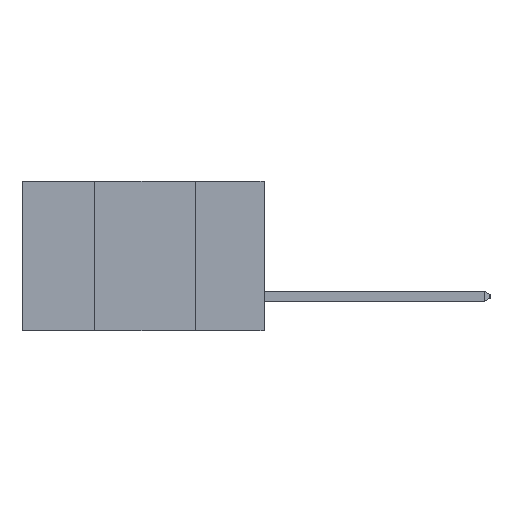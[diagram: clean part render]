
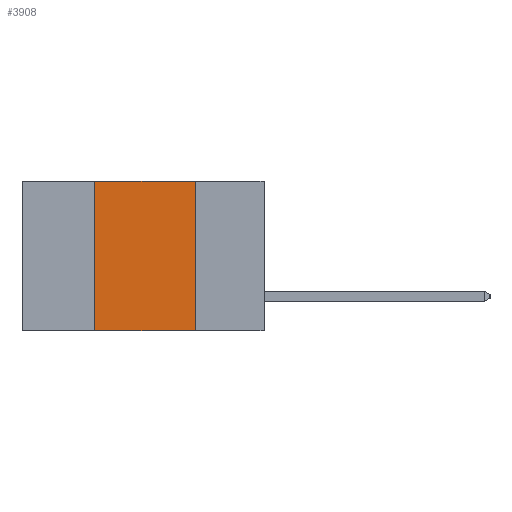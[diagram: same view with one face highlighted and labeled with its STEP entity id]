
A CAD part, left-side view. The second image highlights one B-rep face of the part: STEP entity #3908.
In plain terms, the highlighted planar face has unit normal (-1, 0, 0).
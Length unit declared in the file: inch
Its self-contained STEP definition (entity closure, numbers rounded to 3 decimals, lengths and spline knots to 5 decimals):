
#106 = CARTESIAN_POINT ( 'NONE',  ( 0., 0.6, -0.37 ) ) ;
#1495 = EDGE_LOOP ( 'NONE', ( #17972, #2869, #17055, #5556 ) ) ;
#1849 = CARTESIAN_POINT ( 'NONE',  ( 0., 0.17, 0. ) ) ;
#2804 = VECTOR ( 'NONE', #8386, 39.37008 ) ;
#2869 = ORIENTED_EDGE ( 'NONE', *, *, #15833, .F. ) ;
#3908 = ADVANCED_FACE ( 'NONE', ( #11621 ), #4209, .F. ) ;
#3989 = AXIS2_PLACEMENT_3D ( 'NONE', #4275, #4074, #4058 ) ;
#4058 = DIRECTION ( 'NONE',  ( 0., 0., -1. ) ) ;
#4074 = DIRECTION ( 'NONE',  ( 1., 0., 0. ) ) ;
#4209 = PLANE ( 'NONE',  #3989 ) ;
#4275 = CARTESIAN_POINT ( 'NONE',  ( 0., 0.6, 0. ) ) ;
#4342 = DIRECTION ( 'NONE',  ( 0., 0., 1. ) ) ;
#4562 = EDGE_CURVE ( 'NONE', #18565, #7516, #11821, .T. ) ;
#4950 = VERTEX_POINT ( 'NONE', #15550 ) ;
#5010 = CARTESIAN_POINT ( 'NONE',  ( 0., 0.42, -0.37 ) ) ;
#5436 = CARTESIAN_POINT ( 'NONE',  ( 0., 0.42, -0.37 ) ) ;
#5556 = ORIENTED_EDGE ( 'NONE', *, *, #16079, .T. ) ;
#7516 = VERTEX_POINT ( 'NONE', #8032 ) ;
#8032 = CARTESIAN_POINT ( 'NONE',  ( 0., 0.42, 0. ) ) ;
#8386 = DIRECTION ( 'NONE',  ( 0., 0., -1. ) ) ;
#9040 = CARTESIAN_POINT ( 'NONE',  ( 0., 0.6, 0. ) ) ;
#10104 = VERTEX_POINT ( 'NONE', #1849 ) ;
#10557 = DIRECTION ( 'NONE',  ( 0., -1., 0. ) ) ;
#10886 = EDGE_CURVE ( 'NONE', #10104, #4950, #11085, .T. ) ;
#11085 = LINE ( 'NONE', #17235, #2804 ) ;
#11621 = FACE_OUTER_BOUND ( 'NONE', #1495, .T. ) ;
#11690 = VECTOR ( 'NONE', #15594, 39.37008 ) ;
#11821 = LINE ( 'NONE', #5010, #15264 ) ;
#12162 = LINE ( 'NONE', #106, #11690 ) ;
#15264 = VECTOR ( 'NONE', #4342, 39.37008 ) ;
#15550 = CARTESIAN_POINT ( 'NONE',  ( 0., 0.17, -0.37 ) ) ;
#15594 = DIRECTION ( 'NONE',  ( 0., -1., 0. ) ) ;
#15833 = EDGE_CURVE ( 'NONE', #7516, #10104, #16716, .T. ) ;
#16079 = EDGE_CURVE ( 'NONE', #18565, #4950, #12162, .T. ) ;
#16282 = VECTOR ( 'NONE', #10557, 39.37008 ) ;
#16716 = LINE ( 'NONE', #9040, #16282 ) ;
#17055 = ORIENTED_EDGE ( 'NONE', *, *, #4562, .F. ) ;
#17235 = CARTESIAN_POINT ( 'NONE',  ( 0., 0.17, -0.37 ) ) ;
#17972 = ORIENTED_EDGE ( 'NONE', *, *, #10886, .F. ) ;
#18565 = VERTEX_POINT ( 'NONE', #5436 ) ;
